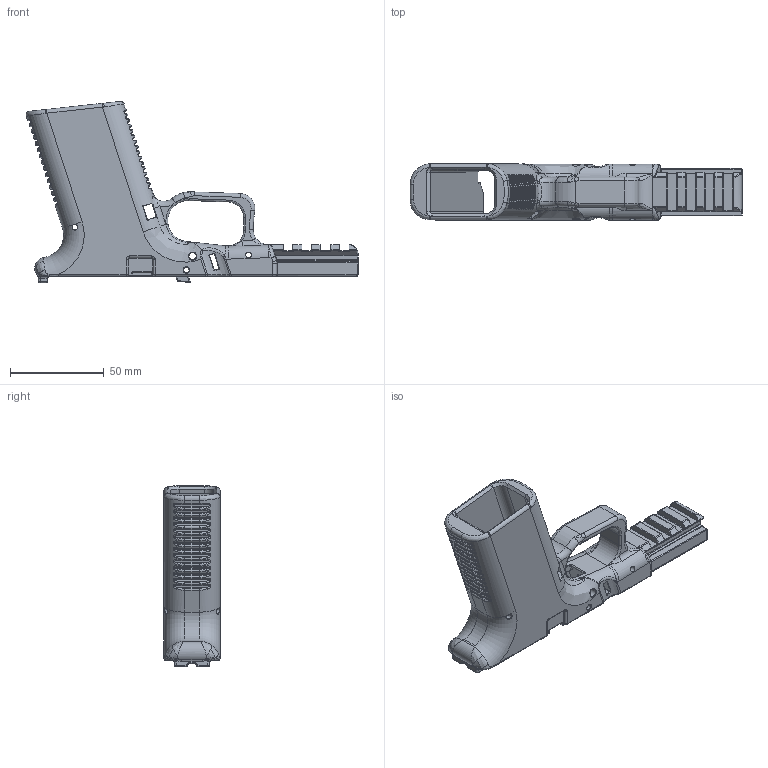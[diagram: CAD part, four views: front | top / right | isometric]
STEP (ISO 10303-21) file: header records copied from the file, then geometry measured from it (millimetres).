
FILE_DESCRIPTION(/* description */ (''),/* implementation_level */ '2;1');
FILE_NAME(/* name */ 'Glock 19 P80.step',/* time_stamp */ '2019-09-18T22:15:33-04:00',/* author */ (''),/* organization */ (''),/* preprocessor_version */ 'ST-DEVELOPER v18',/* originating_system */ 'Autodesk Translation Framework v8.6.0.1094',/* authorisation */ '');
FILE_SCHEMA (('AUTOMOTIVE_DESIGN { 1 0 10303 214 3 1 1 }'));
Products named in the file (1): Glock 19 P80
Bounding box: 177.5 x 30 x 96.84 mm (x, y, z)
Volume: 87079.6 mm3; surface area: 44435.4 mm2
Topology: 1 solids, 1 shells, 1676 faces, 4033 edges, 2269 vertices
Faces by surface type: bspline 571, cylinder 568, plane 287, torus 153, sphere 79, cone 18
Full cylindrical faces by diameter (mm): 2.997 x2, 3 x5, 3.962 x2
Entity records: 65699 total; most frequent: CARTESIAN_POINT 29175, ORIENTED_EDGE 7922, DIRECTION 7337, EDGE_CURVE 3961, AXIS2_PLACEMENT_3D 3006, VERTEX_POINT 2273, EDGE_LOOP 1694, FACE_OUTER_BOUND 1676
